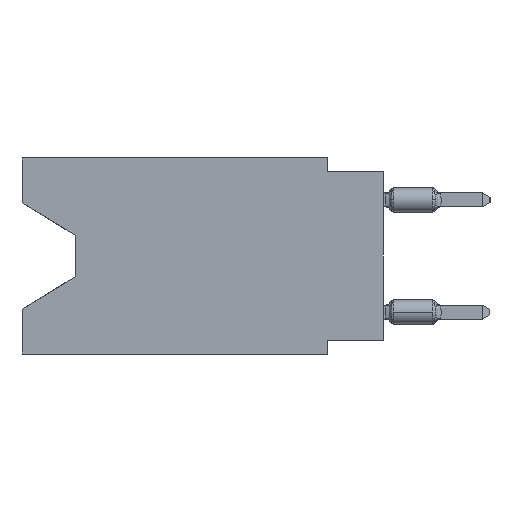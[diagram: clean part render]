
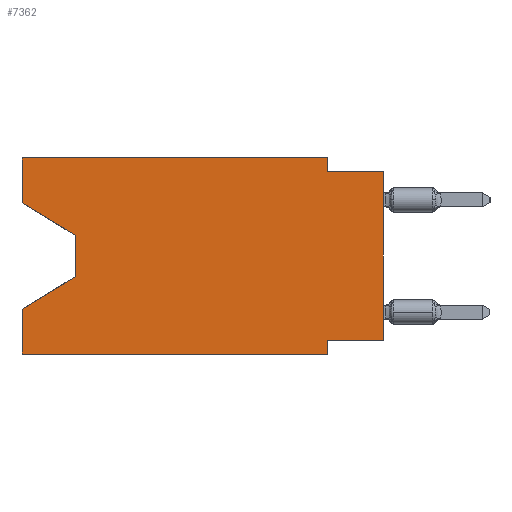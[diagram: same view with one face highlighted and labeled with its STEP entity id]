
A CAD part, left-side view. The second image highlights one B-rep face of the part: STEP entity #7362.
In plain terms, the highlighted planar face has unit normal (-1, 0, 0).
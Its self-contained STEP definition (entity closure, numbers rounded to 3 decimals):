
#253 = VECTOR ( 'NONE', #17743, 1000. ) ;
#400 = VERTEX_POINT ( 'NONE', #15789 ) ;
#406 = VERTEX_POINT ( 'NONE', #13832 ) ;
#969 = LINE ( 'NONE', #20428, #11464 ) ;
#1002 = CARTESIAN_POINT ( 'NONE',  ( 0., 13.97, -5.385 ) ) ;
#2093 = ORIENTED_EDGE ( 'NONE', *, *, #27237, .F. ) ;
#2115 = CARTESIAN_POINT ( 'NONE',  ( 0., 2.54, 0. ) ) ;
#2334 = LINE ( 'NONE', #15329, #10123 ) ;
#2772 = LINE ( 'NONE', #7087, #17934 ) ;
#2912 = VERTEX_POINT ( 'NONE', #16159 ) ;
#3109 = CARTESIAN_POINT ( 'NONE',  ( 0., 16.383, -8.89 ) ) ;
#3681 = EDGE_CURVE ( 'NONE', #22684, #4625, #969, .T. ) ;
#3728 = ORIENTED_EDGE ( 'NONE', *, *, #13112, .F. ) ;
#3741 = ORIENTED_EDGE ( 'NONE', *, *, #27345, .T. ) ;
#3773 = CARTESIAN_POINT ( 'NONE',  ( 0., 16.383, 0. ) ) ;
#4143 = DIRECTION ( 'NONE',  ( 0., 0.855, -0.519 ) ) ;
#4298 = DIRECTION ( 'NONE',  ( 0., 1., 0. ) ) ;
#4433 = AXIS2_PLACEMENT_3D ( 'NONE', #6444, #15401, #15272 ) ;
#4625 = VERTEX_POINT ( 'NONE', #1002 ) ;
#5068 = CARTESIAN_POINT ( 'NONE',  ( 0., 2.54, -8.89 ) ) ;
#5098 = CARTESIAN_POINT ( 'NONE',  ( 0., 0., 0. ) ) ;
#5133 = CARTESIAN_POINT ( 'NONE',  ( 0., 2.54, -8.89 ) ) ;
#6238 = DIRECTION ( 'NONE',  ( 0., 0., 1. ) ) ;
#6264 = CARTESIAN_POINT ( 'NONE',  ( 0., 0., -8.255 ) ) ;
#6300 = ORIENTED_EDGE ( 'NONE', *, *, #23662, .F. ) ;
#6444 = CARTESIAN_POINT ( 'NONE',  ( 0., 16.383, 0. ) ) ;
#6857 = FACE_OUTER_BOUND ( 'NONE', #20493, .T. ) ;
#6913 = CARTESIAN_POINT ( 'NONE',  ( 0., 16.383, -2.038 ) ) ;
#7087 = CARTESIAN_POINT ( 'NONE',  ( 0., 16.383, 0. ) ) ;
#7362 = ADVANCED_FACE ( 'NONE', ( #6857 ), #19480, .F. ) ;
#8068 = VERTEX_POINT ( 'NONE', #20686 ) ;
#8653 = ORIENTED_EDGE ( 'NONE', *, *, #20850, .T. ) ;
#8661 = ORIENTED_EDGE ( 'NONE', *, *, #13712, .F. ) ;
#9778 = DIRECTION ( 'NONE',  ( 0., 0., -1. ) ) ;
#9986 = VERTEX_POINT ( 'NONE', #21092 ) ;
#10065 = DIRECTION ( 'NONE',  ( 0., 0., 1. ) ) ;
#10123 = VECTOR ( 'NONE', #23786, 1000. ) ;
#10323 = VECTOR ( 'NONE', #4143, 1000. ) ;
#11126 = ORIENTED_EDGE ( 'NONE', *, *, #3681, .T. ) ;
#11400 = ORIENTED_EDGE ( 'NONE', *, *, #21273, .T. ) ;
#11464 = VECTOR ( 'NONE', #9778, 1000. ) ;
#12948 = DIRECTION ( 'NONE',  ( 0., -0.855, -0.519 ) ) ;
#13112 = EDGE_CURVE ( 'NONE', #9986, #400, #24975, .T. ) ;
#13632 = DIRECTION ( 'NONE',  ( 0., 0., 1. ) ) ;
#13712 = EDGE_CURVE ( 'NONE', #16456, #20103, #21258, .T. ) ;
#13832 = CARTESIAN_POINT ( 'NONE',  ( 0., 2.54, -0.635 ) ) ;
#13890 = LINE ( 'NONE', #5068, #25961 ) ;
#13947 = CARTESIAN_POINT ( 'NONE',  ( 0., 16.383, -8.89 ) ) ;
#14360 = CARTESIAN_POINT ( 'NONE',  ( 0., 13.97, -5.385 ) ) ;
#15197 = LINE ( 'NONE', #6913, #26989 ) ;
#15272 = DIRECTION ( 'NONE',  ( 0., 0., -1. ) ) ;
#15329 = CARTESIAN_POINT ( 'NONE',  ( 0., 0., -0.635 ) ) ;
#15401 = DIRECTION ( 'NONE',  ( 1., 0., 0. ) ) ;
#15441 = ORIENTED_EDGE ( 'NONE', *, *, #24079, .F. ) ;
#15638 = DIRECTION ( 'NONE',  ( 0., -1., 0. ) ) ;
#15789 = CARTESIAN_POINT ( 'NONE',  ( 0., 16.383, 0. ) ) ;
#15922 = VECTOR ( 'NONE', #10065, 1000. ) ;
#16159 = CARTESIAN_POINT ( 'NONE',  ( 0., 16.383, -6.852 ) ) ;
#16456 = VERTEX_POINT ( 'NONE', #16912 ) ;
#16912 = CARTESIAN_POINT ( 'NONE',  ( 0., 0., -8.255 ) ) ;
#17377 = LINE ( 'NONE', #2115, #25825 ) ;
#17743 = DIRECTION ( 'NONE',  ( 0., -1., 0. ) ) ;
#17934 = VECTOR ( 'NONE', #15638, 1000. ) ;
#18781 = CARTESIAN_POINT ( 'NONE',  ( 0., 2.54, -8.255 ) ) ;
#19413 = ORIENTED_EDGE ( 'NONE', *, *, #22868, .T. ) ;
#19480 = PLANE ( 'NONE',  #4433 ) ;
#20082 = VERTEX_POINT ( 'NONE', #3109 ) ;
#20103 = VERTEX_POINT ( 'NONE', #18781 ) ;
#20169 = VECTOR ( 'NONE', #6238, 1000. ) ;
#20428 = CARTESIAN_POINT ( 'NONE',  ( 0., 13.97, -3.505 ) ) ;
#20493 = EDGE_LOOP ( 'NONE', ( #19413, #11126, #3741, #27026, #8653, #27600, #8661, #11400, #15441, #6300, #2093, #3728 ) ) ;
#20686 = CARTESIAN_POINT ( 'NONE',  ( 0., 0., -0.635 ) ) ;
#20850 = EDGE_CURVE ( 'NONE', #20082, #25492, #26757, .T. ) ;
#21092 = CARTESIAN_POINT ( 'NONE',  ( 0., 16.383, -2.038 ) ) ;
#21177 = VERTEX_POINT ( 'NONE', #24459 ) ;
#21232 = LINE ( 'NONE', #14360, #10323 ) ;
#21258 = LINE ( 'NONE', #6264, #25398 ) ;
#21273 = EDGE_CURVE ( 'NONE', #16456, #8068, #24323, .T. ) ;
#21714 = DIRECTION ( 'NONE',  ( 0., 0., -1. ) ) ;
#21779 = VECTOR ( 'NONE', #13632, 1000. ) ;
#22100 = CARTESIAN_POINT ( 'NONE',  ( 0., 13.97, -3.505 ) ) ;
#22588 = DIRECTION ( 'NONE',  ( 0., 0., -1. ) ) ;
#22684 = VERTEX_POINT ( 'NONE', #22100 ) ;
#22868 = EDGE_CURVE ( 'NONE', #9986, #22684, #15197, .T. ) ;
#23360 = CARTESIAN_POINT ( 'NONE',  ( 0., 16.383, 0. ) ) ;
#23662 = EDGE_CURVE ( 'NONE', #21177, #406, #17377, .T. ) ;
#23786 = DIRECTION ( 'NONE',  ( 0., -1., 0. ) ) ;
#24079 = EDGE_CURVE ( 'NONE', #406, #8068, #2334, .T. ) ;
#24323 = LINE ( 'NONE', #5098, #21779 ) ;
#24459 = CARTESIAN_POINT ( 'NONE',  ( 0., 2.54, 0. ) ) ;
#24975 = LINE ( 'NONE', #3773, #15922 ) ;
#25326 = LINE ( 'NONE', #23360, #20169 ) ;
#25398 = VECTOR ( 'NONE', #4298, 1000. ) ;
#25492 = VERTEX_POINT ( 'NONE', #5133 ) ;
#25816 = EDGE_CURVE ( 'NONE', #20103, #25492, #13890, .T. ) ;
#25825 = VECTOR ( 'NONE', #21714, 1000. ) ;
#25961 = VECTOR ( 'NONE', #22588, 1000. ) ;
#26757 = LINE ( 'NONE', #13947, #253 ) ;
#26989 = VECTOR ( 'NONE', #12948, 1000. ) ;
#27026 = ORIENTED_EDGE ( 'NONE', *, *, #27483, .F. ) ;
#27237 = EDGE_CURVE ( 'NONE', #400, #21177, #2772, .T. ) ;
#27345 = EDGE_CURVE ( 'NONE', #4625, #2912, #21232, .T. ) ;
#27483 = EDGE_CURVE ( 'NONE', #20082, #2912, #25326, .T. ) ;
#27600 = ORIENTED_EDGE ( 'NONE', *, *, #25816, .F. ) ;
